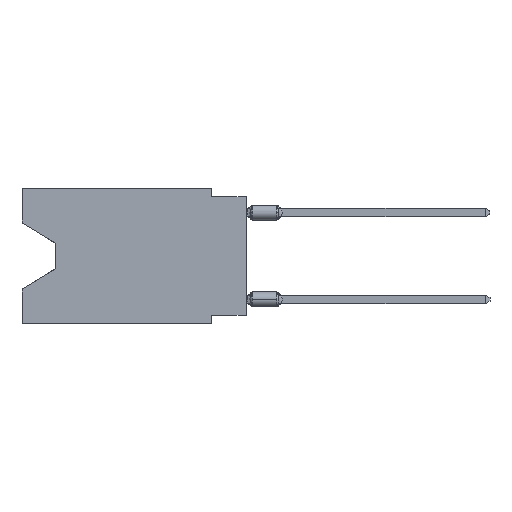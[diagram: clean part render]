
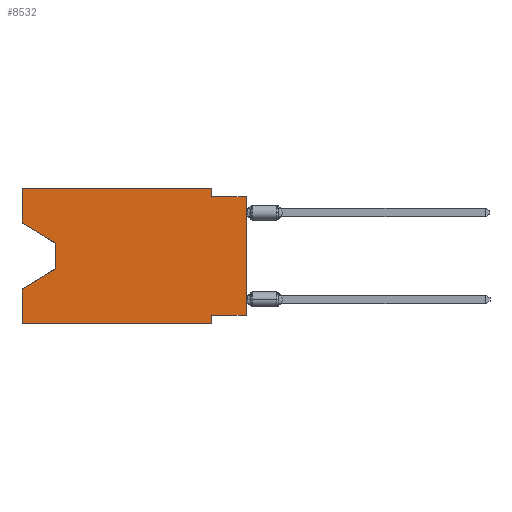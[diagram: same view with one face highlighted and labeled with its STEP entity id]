
A CAD part, left-side view. The second image highlights one B-rep face of the part: STEP entity #8532.
In plain terms, the highlighted planar face has unit normal (-1, 0, 0).
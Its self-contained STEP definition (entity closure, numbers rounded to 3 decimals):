
#197 = CARTESIAN_POINT ( 'NONE',  ( 0., 0., -0.635 ) ) ;
#217 = LINE ( 'NONE', #17894, #22709 ) ;
#293 = DIRECTION ( 'NONE',  ( 0., 0.855, -0.519 ) ) ;
#574 = DIRECTION ( 'NONE',  ( 0., -1., 0. ) ) ;
#903 = DIRECTION ( 'NONE',  ( 0., 0., 1. ) ) ;
#1465 = DIRECTION ( 'NONE',  ( 0., 0., 1. ) ) ;
#2460 = LINE ( 'NONE', #11205, #24839 ) ;
#2675 = DIRECTION ( 'NONE',  ( 0., 0., -1. ) ) ;
#2768 = CARTESIAN_POINT ( 'NONE',  ( 0., 2.54, -9.271 ) ) ;
#3281 = CARTESIAN_POINT ( 'NONE',  ( 0., 16.383, 0. ) ) ;
#3334 = LINE ( 'NONE', #23135, #24136 ) ;
#3808 = EDGE_CURVE ( 'NONE', #9259, #25919, #14100, .T. ) ;
#4668 = DIRECTION ( 'NONE',  ( 0., -1., 0. ) ) ;
#4818 = VERTEX_POINT ( 'NONE', #26239 ) ;
#5359 = DIRECTION ( 'NONE',  ( 0., 1., 0. ) ) ;
#7027 = CARTESIAN_POINT ( 'NONE',  ( 0., 16.383, -2.546 ) ) ;
#7629 = DIRECTION ( 'NONE',  ( 0., 0., -1. ) ) ;
#7648 = EDGE_CURVE ( 'NONE', #13083, #25173, #12052, .T. ) ;
#7936 = CARTESIAN_POINT ( 'NONE',  ( 0., 16.383, 0. ) ) ;
#8264 = VECTOR ( 'NONE', #7629, 1000. ) ;
#8284 = CARTESIAN_POINT ( 'NONE',  ( 0., 0., 0. ) ) ;
#8382 = CARTESIAN_POINT ( 'NONE',  ( 0., 16.383, 0. ) ) ;
#8532 = ADVANCED_FACE ( 'NONE', ( #18327 ), #9424, .F. ) ;
#8950 = EDGE_CURVE ( 'NONE', #20061, #11534, #15574, .T. ) ;
#9259 = VERTEX_POINT ( 'NONE', #9467 ) ;
#9312 = DIRECTION ( 'NONE',  ( 0., -0.855, -0.519 ) ) ;
#9316 = ORIENTED_EDGE ( 'NONE', *, *, #26969, .F. ) ;
#9403 = CARTESIAN_POINT ( 'NONE',  ( 0., 2.54, -0.635 ) ) ;
#9424 = PLANE ( 'NONE',  #27811 ) ;
#9467 = CARTESIAN_POINT ( 'NONE',  ( 0., 13.97, -4.013 ) ) ;
#10176 = VECTOR ( 'NONE', #20711, 1000. ) ;
#10765 = VECTOR ( 'NONE', #4668, 1000. ) ;
#11205 = CARTESIAN_POINT ( 'NONE',  ( 0., 13.97, -5.893 ) ) ;
#11477 = EDGE_CURVE ( 'NONE', #25173, #12627, #11533, .T. ) ;
#11534 = VERTEX_POINT ( 'NONE', #26915 ) ;
#11533 = LINE ( 'NONE', #197, #18220 ) ;
#11637 = VERTEX_POINT ( 'NONE', #22600 ) ;
#12052 = LINE ( 'NONE', #13777, #8264 ) ;
#12367 = LINE ( 'NONE', #21127, #25907 ) ;
#12564 = LINE ( 'NONE', #8284, #22755 ) ;
#12627 = VERTEX_POINT ( 'NONE', #14761 ) ;
#13083 = VERTEX_POINT ( 'NONE', #19849 ) ;
#13214 = LINE ( 'NONE', #3281, #24701 ) ;
#13400 = DIRECTION ( 'NONE',  ( 0., -1., 0. ) ) ;
#13777 = CARTESIAN_POINT ( 'NONE',  ( 0., 2.54, 0. ) ) ;
#14100 = LINE ( 'NONE', #22875, #10176 ) ;
#14761 = CARTESIAN_POINT ( 'NONE',  ( 0., 0., -0.635 ) ) ;
#14810 = EDGE_CURVE ( 'NONE', #25919, #4818, #2460, .T. ) ;
#14920 = VECTOR ( 'NONE', #9312, 1000. ) ;
#15574 = LINE ( 'NONE', #24325, #10765 ) ;
#16686 = ORIENTED_EDGE ( 'NONE', *, *, #25084, .T. ) ;
#17287 = ORIENTED_EDGE ( 'NONE', *, *, #3808, .T. ) ;
#17311 = DIRECTION ( 'NONE',  ( 0., 0., 1. ) ) ;
#17642 = CARTESIAN_POINT ( 'NONE',  ( 0., 16.383, -2.546 ) ) ;
#17894 = CARTESIAN_POINT ( 'NONE',  ( 0., 2.54, -9.906 ) ) ;
#18183 = DIRECTION ( 'NONE',  ( 1., 0., 0. ) ) ;
#18220 = VECTOR ( 'NONE', #13400, 1000. ) ;
#18327 = FACE_OUTER_BOUND ( 'NONE', #25277, .T. ) ;
#18674 = CARTESIAN_POINT ( 'NONE',  ( 0., 16.383, -9.906 ) ) ;
#18696 = LINE ( 'NONE', #7936, #28255 ) ;
#18771 = ORIENTED_EDGE ( 'NONE', *, *, #14810, .T. ) ;
#19828 = CARTESIAN_POINT ( 'NONE',  ( 0., 13.97, -5.893 ) ) ;
#19849 = CARTESIAN_POINT ( 'NONE',  ( 0., 2.54, 0. ) ) ;
#20052 = CARTESIAN_POINT ( 'NONE',  ( 0., 16.383, 0. ) ) ;
#20061 = VERTEX_POINT ( 'NONE', #18674 ) ;
#20711 = DIRECTION ( 'NONE',  ( 0., 0., -1. ) ) ;
#20802 = VERTEX_POINT ( 'NONE', #7027 ) ;
#21127 = CARTESIAN_POINT ( 'NONE',  ( 0., 16.383, 0. ) ) ;
#21726 = EDGE_CURVE ( 'NONE', #26629, #13083, #13214, .T. ) ;
#22079 = ORIENTED_EDGE ( 'NONE', *, *, #11477, .F. ) ;
#22600 = CARTESIAN_POINT ( 'NONE',  ( 0., 0., -9.271 ) ) ;
#22709 = VECTOR ( 'NONE', #2675, 1000. ) ;
#22755 = VECTOR ( 'NONE', #17311, 1000. ) ;
#22875 = CARTESIAN_POINT ( 'NONE',  ( 0., 13.97, -4.013 ) ) ;
#23135 = CARTESIAN_POINT ( 'NONE',  ( 0., 0., -9.271 ) ) ;
#23308 = ORIENTED_EDGE ( 'NONE', *, *, #7648, .F. ) ;
#23496 = VERTEX_POINT ( 'NONE', #2768 ) ;
#24086 = EDGE_CURVE ( 'NONE', #23496, #11534, #217, .T. ) ;
#24136 = VECTOR ( 'NONE', #5359, 1000. ) ;
#24325 = CARTESIAN_POINT ( 'NONE',  ( 0., 16.383, -9.906 ) ) ;
#24361 = ORIENTED_EDGE ( 'NONE', *, *, #21726, .F. ) ;
#24701 = VECTOR ( 'NONE', #574, 1000. ) ;
#24839 = VECTOR ( 'NONE', #293, 1000. ) ;
#25084 = EDGE_CURVE ( 'NONE', #11637, #12627, #12564, .T. ) ;
#25173 = VERTEX_POINT ( 'NONE', #9403 ) ;
#25183 = ORIENTED_EDGE ( 'NONE', *, *, #25727, .F. ) ;
#25277 = EDGE_LOOP ( 'NONE', ( #26961, #17287, #18771, #9316, #25488, #26355, #25183, #16686, #22079, #23308, #24361, #27114 ) ) ;
#25488 = ORIENTED_EDGE ( 'NONE', *, *, #8950, .T. ) ;
#25727 = EDGE_CURVE ( 'NONE', #11637, #23496, #3334, .T. ) ;
#25907 = VECTOR ( 'NONE', #1465, 1000. ) ;
#25919 = VERTEX_POINT ( 'NONE', #19828 ) ;
#26239 = CARTESIAN_POINT ( 'NONE',  ( 0., 16.383, -7.36 ) ) ;
#26355 = ORIENTED_EDGE ( 'NONE', *, *, #24086, .F. ) ;
#26629 = VERTEX_POINT ( 'NONE', #8382 ) ;
#26695 = LINE ( 'NONE', #17642, #14920 ) ;
#26915 = CARTESIAN_POINT ( 'NONE',  ( 0., 2.54, -9.906 ) ) ;
#26951 = DIRECTION ( 'NONE',  ( 0., 0., -1. ) ) ;
#26961 = ORIENTED_EDGE ( 'NONE', *, *, #27743, .T. ) ;
#26969 = EDGE_CURVE ( 'NONE', #20061, #4818, #18696, .T. ) ;
#27090 = EDGE_CURVE ( 'NONE', #20802, #26629, #12367, .T. ) ;
#27114 = ORIENTED_EDGE ( 'NONE', *, *, #27090, .F. ) ;
#27743 = EDGE_CURVE ( 'NONE', #20802, #9259, #26695, .T. ) ;
#27811 = AXIS2_PLACEMENT_3D ( 'NONE', #20052, #18183, #26951 ) ;
#28255 = VECTOR ( 'NONE', #903, 1000. ) ;
